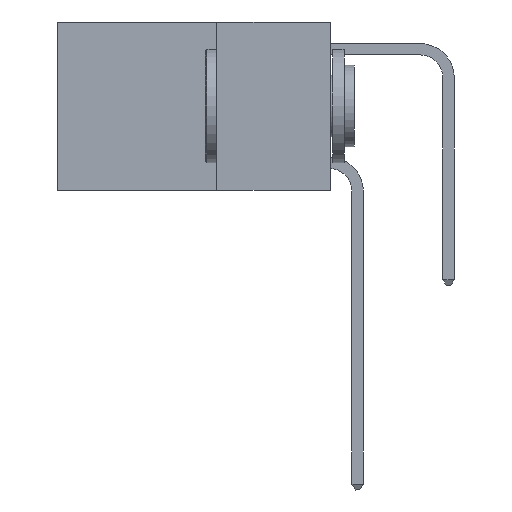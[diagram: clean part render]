
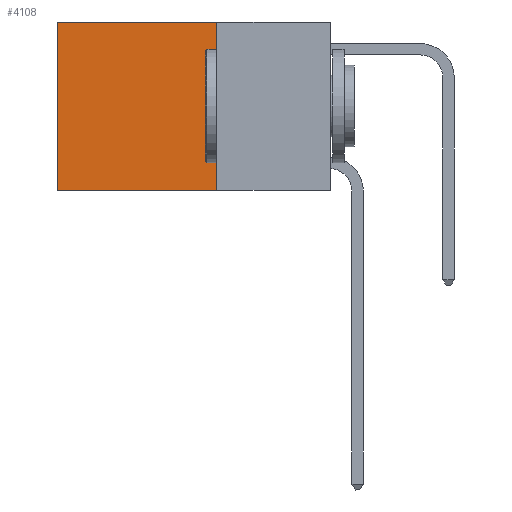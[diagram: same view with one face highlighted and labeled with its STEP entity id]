
A CAD part, left-side view. The second image highlights one B-rep face of the part: STEP entity #4108.
In plain terms, the highlighted planar face has unit normal (-1, 0, 0).
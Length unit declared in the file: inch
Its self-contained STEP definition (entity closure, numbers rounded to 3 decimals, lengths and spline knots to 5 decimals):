
#361 = CARTESIAN_POINT ( 'NONE',  ( 0.2625, 0.6, 0. ) ) ;
#661 = LINE ( 'NONE', #7436, #9844 ) ;
#683 = EDGE_CURVE ( 'NONE', #6450, #2761, #661, .T. ) ;
#812 = EDGE_CURVE ( 'NONE', #2236, #9375, #3898, .T. ) ;
#962 = DIRECTION ( 'NONE',  ( 0., 0., -1. ) ) ;
#1070 = DIRECTION ( 'NONE',  ( 1., 0., 0. ) ) ;
#1083 = CARTESIAN_POINT ( 'NONE',  ( 0.2625, 0.25, 0. ) ) ;
#1153 = PLANE ( 'NONE',  #10418 ) ;
#1603 = VECTOR ( 'NONE', #5687, 39.37008 ) ;
#1689 = VECTOR ( 'NONE', #8538, 39.37008 ) ;
#1802 = CARTESIAN_POINT ( 'NONE',  ( 0.2625, 0.6, 0. ) ) ;
#2236 = VERTEX_POINT ( 'NONE', #3178 ) ;
#2761 = VERTEX_POINT ( 'NONE', #361 ) ;
#3177 = ORIENTED_EDGE ( 'NONE', *, *, #683, .T. ) ;
#3178 = CARTESIAN_POINT ( 'NONE',  ( 0.2625, 0.25, -0.37 ) ) ;
#3555 = EDGE_CURVE ( 'NONE', #2761, #9375, #10057, .T. ) ;
#3751 = ORIENTED_EDGE ( 'NONE', *, *, #3555, .T. ) ;
#3756 = CARTESIAN_POINT ( 'NONE',  ( 0.2625, 0.6, -0.37 ) ) ;
#3898 = LINE ( 'NONE', #10425, #1603 ) ;
#3916 = ORIENTED_EDGE ( 'NONE', *, *, #812, .F. ) ;
#4108 = ADVANCED_FACE ( 'NONE', ( #6791 ), #1153, .F. ) ;
#4401 = VECTOR ( 'NONE', #5736, 39.37008 ) ;
#4612 = ORIENTED_EDGE ( 'NONE', *, *, #4766, .F. ) ;
#4766 = EDGE_CURVE ( 'NONE', #6450, #2236, #10881, .T. ) ;
#5588 = CARTESIAN_POINT ( 'NONE',  ( 0.2625, 0.25, 0. ) ) ;
#5687 = DIRECTION ( 'NONE',  ( 0., 1., 0. ) ) ;
#5736 = DIRECTION ( 'NONE',  ( 0., 0., -1. ) ) ;
#5791 = CARTESIAN_POINT ( 'NONE',  ( 0.2625, 0.25, 0. ) ) ;
#6450 = VERTEX_POINT ( 'NONE', #5588 ) ;
#6791 = FACE_OUTER_BOUND ( 'NONE', #7103, .T. ) ;
#7103 = EDGE_LOOP ( 'NONE', ( #3751, #3916, #4612, #3177 ) ) ;
#7436 = CARTESIAN_POINT ( 'NONE',  ( 0.2625, 0.25, 0. ) ) ;
#8538 = DIRECTION ( 'NONE',  ( 0., 0., -1. ) ) ;
#9328 = DIRECTION ( 'NONE',  ( 0., 1., 0. ) ) ;
#9375 = VERTEX_POINT ( 'NONE', #3756 ) ;
#9844 = VECTOR ( 'NONE', #9328, 39.37008 ) ;
#10057 = LINE ( 'NONE', #1802, #1689 ) ;
#10418 = AXIS2_PLACEMENT_3D ( 'NONE', #1083, #1070, #962 ) ;
#10425 = CARTESIAN_POINT ( 'NONE',  ( 0.2625, 0.25, -0.37 ) ) ;
#10881 = LINE ( 'NONE', #5791, #4401 ) ;
